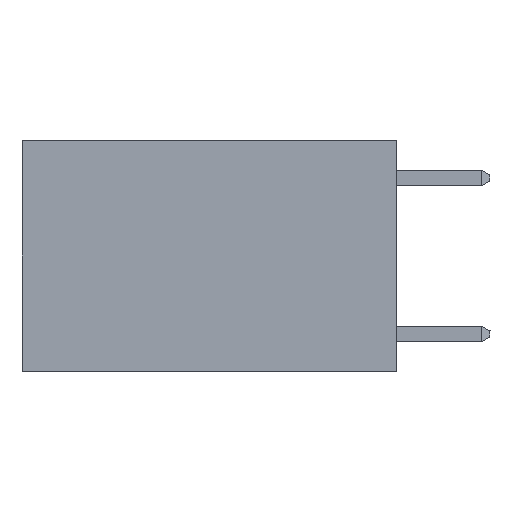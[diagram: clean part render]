
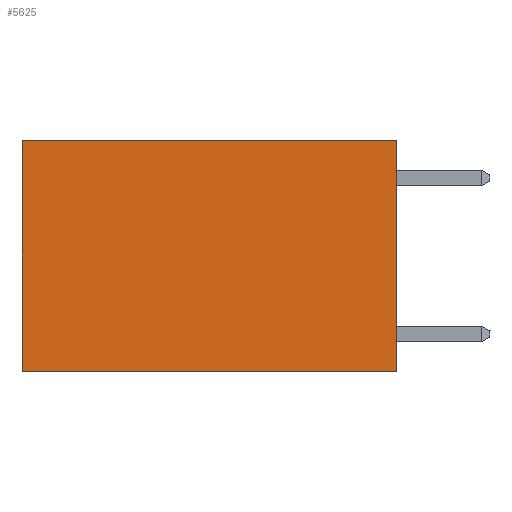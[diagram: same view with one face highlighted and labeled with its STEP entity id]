
A CAD part, left-side view. The second image highlights one B-rep face of the part: STEP entity #5625.
In plain terms, the highlighted planar face has unit normal (-1, 0, 0).
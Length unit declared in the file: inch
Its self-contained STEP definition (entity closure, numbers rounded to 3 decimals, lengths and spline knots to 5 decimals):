
#36 = VECTOR ( 'NONE', #6827, 39.37008 ) ;
#149 = DIRECTION ( 'NONE',  ( 0., 0., -1. ) ) ;
#1129 = EDGE_CURVE ( 'NONE', #24477, #19787, #18489, .T. ) ;
#1492 = ORIENTED_EDGE ( 'NONE', *, *, #10337, .F. ) ;
#2062 = AXIS2_PLACEMENT_3D ( 'NONE', #11832, #14316, #29513 ) ;
#2486 = CARTESIAN_POINT ( 'NONE',  ( 0.2625, 0., 0. ) ) ;
#2853 = CARTESIAN_POINT ( 'NONE',  ( 0.2625, 0., 0. ) ) ;
#5093 = CARTESIAN_POINT ( 'NONE',  ( 0.2625, 0., -0.37 ) ) ;
#5625 = ADVANCED_FACE ( 'NONE', ( #27203 ), #11940, .F. ) ;
#5997 = CARTESIAN_POINT ( 'NONE',  ( 0.2625, 0.6, -0.37 ) ) ;
#6212 = CARTESIAN_POINT ( 'NONE',  ( 0.2625, 0.6, 0. ) ) ;
#6827 = DIRECTION ( 'NONE',  ( 0., 0., -1. ) ) ;
#7315 = DIRECTION ( 'NONE',  ( 0., 1., 0. ) ) ;
#8306 = EDGE_CURVE ( 'NONE', #25570, #24477, #24523, .T. ) ;
#8484 = VECTOR ( 'NONE', #149, 39.37008 ) ;
#10337 = EDGE_CURVE ( 'NONE', #25164, #19787, #30576, .T. ) ;
#11739 = VECTOR ( 'NONE', #17024, 39.37008 ) ;
#11831 = EDGE_LOOP ( 'NONE', ( #13242, #1492, #18545, #16927 ) ) ;
#11832 = CARTESIAN_POINT ( 'NONE',  ( 0.2625, 0., 0. ) ) ;
#11940 = PLANE ( 'NONE',  #2062 ) ;
#12557 = VECTOR ( 'NONE', #7315, 39.37008 ) ;
#13242 = ORIENTED_EDGE ( 'NONE', *, *, #1129, .T. ) ;
#14316 = DIRECTION ( 'NONE',  ( 1., 0., 0. ) ) ;
#16927 = ORIENTED_EDGE ( 'NONE', *, *, #8306, .T. ) ;
#17024 = DIRECTION ( 'NONE',  ( 0., 1., 0. ) ) ;
#18095 = CARTESIAN_POINT ( 'NONE',  ( 0.2625, 0., -0.37 ) ) ;
#18489 = LINE ( 'NONE', #20250, #36 ) ;
#18545 = ORIENTED_EDGE ( 'NONE', *, *, #21000, .F. ) ;
#19787 = VERTEX_POINT ( 'NONE', #5997 ) ;
#20250 = CARTESIAN_POINT ( 'NONE',  ( 0.2625, 0.6, 0. ) ) ;
#21000 = EDGE_CURVE ( 'NONE', #25570, #25164, #21955, .T. ) ;
#21610 = CARTESIAN_POINT ( 'NONE',  ( 0.2625, 0., 0. ) ) ;
#21955 = LINE ( 'NONE', #2486, #8484 ) ;
#24477 = VERTEX_POINT ( 'NONE', #6212 ) ;
#24523 = LINE ( 'NONE', #21610, #12557 ) ;
#25164 = VERTEX_POINT ( 'NONE', #18095 ) ;
#25570 = VERTEX_POINT ( 'NONE', #2853 ) ;
#27203 = FACE_OUTER_BOUND ( 'NONE', #11831, .T. ) ;
#29513 = DIRECTION ( 'NONE',  ( 0., 0., -1. ) ) ;
#30576 = LINE ( 'NONE', #5093, #11739 ) ;
